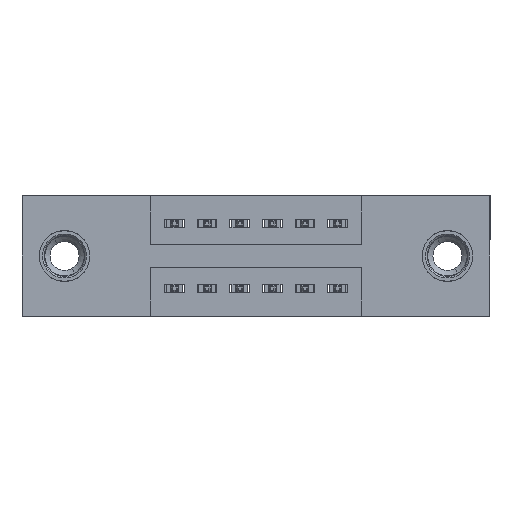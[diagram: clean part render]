
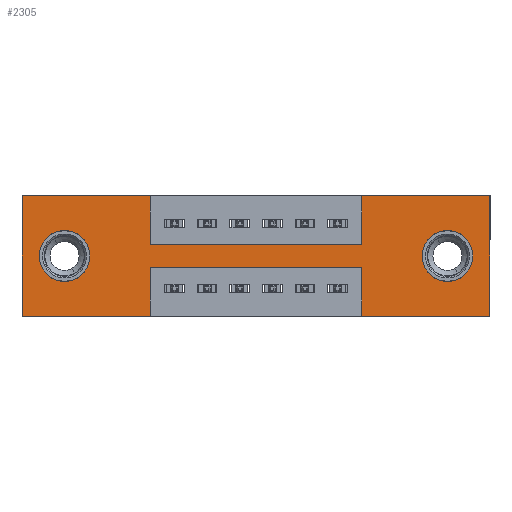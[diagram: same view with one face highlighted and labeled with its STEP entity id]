
A CAD part, front view. The second image highlights one B-rep face of the part: STEP entity #2305.
In plain terms, the highlighted planar face has unit normal (0, -1, 0).
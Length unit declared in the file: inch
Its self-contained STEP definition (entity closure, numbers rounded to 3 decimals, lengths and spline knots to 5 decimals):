
#58 = EDGE_CURVE ( 'NONE', #11622, #13202, #197, .T. ) ;
#131 = CARTESIAN_POINT ( 'NONE',  ( 0.3925, 0., -0.15 ) ) ;
#153 = VECTOR ( 'NONE', #11398, 39.37008 ) ;
#197 = LINE ( 'NONE', #3537, #5478 ) ;
#442 = AXIS2_PLACEMENT_3D ( 'NONE', #4278, #12115, #5406 ) ;
#526 = AXIS2_PLACEMENT_3D ( 'NONE', #6575, #14260, #7743 ) ;
#680 = CARTESIAN_POINT ( 'NONE',  ( 1.0425, 0., -0.22 ) ) ;
#796 = EDGE_CURVE ( 'NONE', #10168, #9665, #11287, .T. ) ;
#981 = CIRCLE ( 'NONE', #526, 0.078 ) ;
#1127 = DIRECTION ( 'NONE',  ( -1., 0., 0. ) ) ;
#1456 = VERTEX_POINT ( 'NONE', #1657 ) ;
#1501 = LINE ( 'NONE', #12642, #1856 ) ;
#1534 = FACE_BOUND ( 'NONE', #10932, .T. ) ;
#1574 = VERTEX_POINT ( 'NONE', #4336 ) ;
#1594 = VERTEX_POINT ( 'NONE', #11284 ) ;
#1657 = CARTESIAN_POINT ( 'NONE',  ( 0.13, 0., -0.107 ) ) ;
#1856 = VECTOR ( 'NONE', #9416, 39.37008 ) ;
#2087 = AXIS2_PLACEMENT_3D ( 'NONE', #6270, #10856, #6394 ) ;
#2255 = VERTEX_POINT ( 'NONE', #2489 ) ;
#2305 = ADVANCED_FACE ( 'NONE', ( #7554, #1534, #13073 ), #7007, .T. ) ;
#2447 = CARTESIAN_POINT ( 'NONE',  ( 1.0425, 0., -0.37 ) ) ;
#2489 = CARTESIAN_POINT ( 'NONE',  ( 1.0425, 0., 0. ) ) ;
#2620 = VECTOR ( 'NONE', #13162, 39.37008 ) ;
#2653 = VECTOR ( 'NONE', #12266, 39.37008 ) ;
#2671 = CARTESIAN_POINT ( 'NONE',  ( 0.3925, 0., 0. ) ) ;
#2856 = EDGE_CURVE ( 'NONE', #12133, #5087, #10217, .T. ) ;
#2940 = CARTESIAN_POINT ( 'NONE',  ( 0., 0., 0. ) ) ;
#3176 = LINE ( 'NONE', #131, #153 ) ;
#3205 = ORIENTED_EDGE ( 'NONE', *, *, #13915, .T. ) ;
#3243 = DIRECTION ( 'NONE',  ( 0., 0., -1. ) ) ;
#3462 = CIRCLE ( 'NONE', #10343, 0.078 ) ;
#3487 = CARTESIAN_POINT ( 'NONE',  ( 0.3925, 0., -0.22 ) ) ;
#3537 = CARTESIAN_POINT ( 'NONE',  ( 0.3925, 0., -0.37 ) ) ;
#3847 = ORIENTED_EDGE ( 'NONE', *, *, #7843, .T. ) ;
#3853 = ORIENTED_EDGE ( 'NONE', *, *, #12224, .F. ) ;
#4213 = VERTEX_POINT ( 'NONE', #2447 ) ;
#4278 = CARTESIAN_POINT ( 'NONE',  ( 0.13, 0., -0.185 ) ) ;
#4336 = CARTESIAN_POINT ( 'NONE',  ( 1.305, 0., -0.263 ) ) ;
#4510 = CARTESIAN_POINT ( 'NONE',  ( 0.3925, 0., 0. ) ) ;
#4565 = CARTESIAN_POINT ( 'NONE',  ( 0.13, 0., -0.185 ) ) ;
#4644 = CARTESIAN_POINT ( 'NONE',  ( 1.0425, 0., 0. ) ) ;
#4929 = VECTOR ( 'NONE', #7155, 39.37008 ) ;
#4982 = CARTESIAN_POINT ( 'NONE',  ( 0.3925, 0., -0.37 ) ) ;
#5003 = AXIS2_PLACEMENT_3D ( 'NONE', #5495, #13262, #6641 ) ;
#5040 = EDGE_CURVE ( 'NONE', #9753, #12133, #5822, .T. ) ;
#5087 = VERTEX_POINT ( 'NONE', #13335 ) ;
#5277 = LINE ( 'NONE', #6020, #4929 ) ;
#5338 = EDGE_CURVE ( 'NONE', #9665, #4213, #5277, .T. ) ;
#5346 = VECTOR ( 'NONE', #10939, 39.37008 ) ;
#5391 = CARTESIAN_POINT ( 'NONE',  ( 0., 0., 0. ) ) ;
#5406 = DIRECTION ( 'NONE',  ( 0., 0., 1. ) ) ;
#5444 = ORIENTED_EDGE ( 'NONE', *, *, #2856, .F. ) ;
#5456 = VECTOR ( 'NONE', #8904, 39.37008 ) ;
#5459 = EDGE_LOOP ( 'NONE', ( #9724, #6595, #9728, #7973, #9478, #6208, #13487, #3853, #5444, #10399, #14210, #7817 ) ) ;
#5478 = VECTOR ( 'NONE', #3243, 39.37008 ) ;
#5495 = CARTESIAN_POINT ( 'NONE',  ( 1.305, 0., -0.185 ) ) ;
#5575 = EDGE_LOOP ( 'NONE', ( #3205, #3847 ) ) ;
#5704 = DIRECTION ( 'NONE',  ( 0., 0., 1. ) ) ;
#5822 = LINE ( 'NONE', #14291, #5456 ) ;
#6020 = CARTESIAN_POINT ( 'NONE',  ( 0., 0., -0.37 ) ) ;
#6204 = ORIENTED_EDGE ( 'NONE', *, *, #14019, .T. ) ;
#6208 = ORIENTED_EDGE ( 'NONE', *, *, #8036, .F. ) ;
#6270 = CARTESIAN_POINT ( 'NONE',  ( 0., 0., -0.37 ) ) ;
#6349 = EDGE_CURVE ( 'NONE', #13573, #9753, #14401, .T. ) ;
#6394 = DIRECTION ( 'NONE',  ( 0., 0., -1. ) ) ;
#6555 = DIRECTION ( 'NONE',  ( 0., 0., -1. ) ) ;
#6575 = CARTESIAN_POINT ( 'NONE',  ( 1.305, 0., -0.185 ) ) ;
#6595 = ORIENTED_EDGE ( 'NONE', *, *, #12988, .F. ) ;
#6641 = DIRECTION ( 'NONE',  ( 0., 0., -1. ) ) ;
#6761 = CARTESIAN_POINT ( 'NONE',  ( 0., 0., -0.37 ) ) ;
#7007 = PLANE ( 'NONE',  #2087 ) ;
#7155 = DIRECTION ( 'NONE',  ( -1., 0., 0. ) ) ;
#7178 = VECTOR ( 'NONE', #6555, 39.37008 ) ;
#7264 = CARTESIAN_POINT ( 'NONE',  ( 1.435, 0., -0.37 ) ) ;
#7554 = FACE_BOUND ( 'NONE', #5575, .T. ) ;
#7743 = DIRECTION ( 'NONE',  ( 0., 0., -1. ) ) ;
#7817 = ORIENTED_EDGE ( 'NONE', *, *, #13548, .F. ) ;
#7843 = EDGE_CURVE ( 'NONE', #1574, #13257, #981, .T. ) ;
#7917 = VECTOR ( 'NONE', #12425, 39.37008 ) ;
#7961 = CARTESIAN_POINT ( 'NONE',  ( 1.435, 0., 0. ) ) ;
#7964 = ORIENTED_EDGE ( 'NONE', *, *, #8695, .T. ) ;
#7973 = ORIENTED_EDGE ( 'NONE', *, *, #5338, .F. ) ;
#8036 = EDGE_CURVE ( 'NONE', #2255, #10168, #1501, .T. ) ;
#8241 = CIRCLE ( 'NONE', #5003, 0.078 ) ;
#8695 = EDGE_CURVE ( 'NONE', #12721, #1456, #14172, .T. ) ;
#8721 = CARTESIAN_POINT ( 'NONE',  ( 1.0425, 0., -0.37 ) ) ;
#8904 = DIRECTION ( 'NONE',  ( 1., 0., 0. ) ) ;
#9176 = VERTEX_POINT ( 'NONE', #680 ) ;
#9268 = EDGE_CURVE ( 'NONE', #4213, #9176, #11345, .T. ) ;
#9416 = DIRECTION ( 'NONE',  ( 1., 0., 0. ) ) ;
#9478 = ORIENTED_EDGE ( 'NONE', *, *, #796, .F. ) ;
#9642 = CARTESIAN_POINT ( 'NONE',  ( 1.435, 0., 0. ) ) ;
#9665 = VERTEX_POINT ( 'NONE', #7264 ) ;
#9724 = ORIENTED_EDGE ( 'NONE', *, *, #58, .F. ) ;
#9728 = ORIENTED_EDGE ( 'NONE', *, *, #9268, .F. ) ;
#9753 = VERTEX_POINT ( 'NONE', #2940 ) ;
#9857 = LINE ( 'NONE', #6761, #12720 ) ;
#10054 = VECTOR ( 'NONE', #11338, 39.37008 ) ;
#10168 = VERTEX_POINT ( 'NONE', #9642 ) ;
#10202 = CARTESIAN_POINT ( 'NONE',  ( 0., 0., -0.37 ) ) ;
#10217 = LINE ( 'NONE', #2671, #7178 ) ;
#10289 = CARTESIAN_POINT ( 'NONE',  ( 0.3925, 0., -0.22 ) ) ;
#10343 = AXIS2_PLACEMENT_3D ( 'NONE', #4565, #12388, #5704 ) ;
#10399 = ORIENTED_EDGE ( 'NONE', *, *, #5040, .F. ) ;
#10856 = DIRECTION ( 'NONE',  ( 0., -1., 0. ) ) ;
#10932 = EDGE_LOOP ( 'NONE', ( #6204, #7964 ) ) ;
#10939 = DIRECTION ( 'NONE',  ( 0., 0., 1. ) ) ;
#11237 = LINE ( 'NONE', #3487, #7917 ) ;
#11284 = CARTESIAN_POINT ( 'NONE',  ( 1.0425, 0., -0.15 ) ) ;
#11287 = LINE ( 'NONE', #7961, #2653 ) ;
#11338 = DIRECTION ( 'NONE',  ( 0., 0., 1. ) ) ;
#11345 = LINE ( 'NONE', #8721, #5346 ) ;
#11398 = DIRECTION ( 'NONE',  ( 1., 0., 0. ) ) ;
#11622 = VERTEX_POINT ( 'NONE', #10289 ) ;
#12115 = DIRECTION ( 'NONE',  ( 0., 1., 0. ) ) ;
#12133 = VERTEX_POINT ( 'NONE', #4510 ) ;
#12224 = EDGE_CURVE ( 'NONE', #5087, #1594, #3176, .T. ) ;
#12266 = DIRECTION ( 'NONE',  ( 0., 0., -1. ) ) ;
#12388 = DIRECTION ( 'NONE',  ( 0., 1., 0. ) ) ;
#12425 = DIRECTION ( 'NONE',  ( -1., 0., 0. ) ) ;
#12642 = CARTESIAN_POINT ( 'NONE',  ( 0., 0., 0. ) ) ;
#12720 = VECTOR ( 'NONE', #1127, 39.37008 ) ;
#12721 = VERTEX_POINT ( 'NONE', #14292 ) ;
#12818 = EDGE_CURVE ( 'NONE', #1594, #2255, #12906, .T. ) ;
#12906 = LINE ( 'NONE', #4644, #10054 ) ;
#12988 = EDGE_CURVE ( 'NONE', #9176, #11622, #11237, .T. ) ;
#13073 = FACE_OUTER_BOUND ( 'NONE', #5459, .T. ) ;
#13162 = DIRECTION ( 'NONE',  ( 0., 0., 1. ) ) ;
#13202 = VERTEX_POINT ( 'NONE', #4982 ) ;
#13257 = VERTEX_POINT ( 'NONE', #13894 ) ;
#13262 = DIRECTION ( 'NONE',  ( 0., 1., 0. ) ) ;
#13335 = CARTESIAN_POINT ( 'NONE',  ( 0.3925, 0., -0.15 ) ) ;
#13487 = ORIENTED_EDGE ( 'NONE', *, *, #12818, .F. ) ;
#13548 = EDGE_CURVE ( 'NONE', #13202, #13573, #9857, .T. ) ;
#13573 = VERTEX_POINT ( 'NONE', #10202 ) ;
#13894 = CARTESIAN_POINT ( 'NONE',  ( 1.305, 0., -0.107 ) ) ;
#13915 = EDGE_CURVE ( 'NONE', #13257, #1574, #8241, .T. ) ;
#14019 = EDGE_CURVE ( 'NONE', #1456, #12721, #3462, .T. ) ;
#14172 = CIRCLE ( 'NONE', #442, 0.078 ) ;
#14210 = ORIENTED_EDGE ( 'NONE', *, *, #6349, .F. ) ;
#14260 = DIRECTION ( 'NONE',  ( 0., 1., 0. ) ) ;
#14291 = CARTESIAN_POINT ( 'NONE',  ( 0., 0., 0. ) ) ;
#14292 = CARTESIAN_POINT ( 'NONE',  ( 0.13, 0., -0.263 ) ) ;
#14401 = LINE ( 'NONE', #5391, #2620 ) ;
